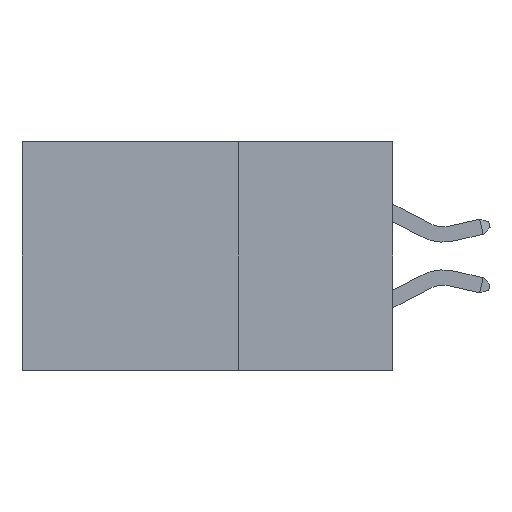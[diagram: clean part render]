
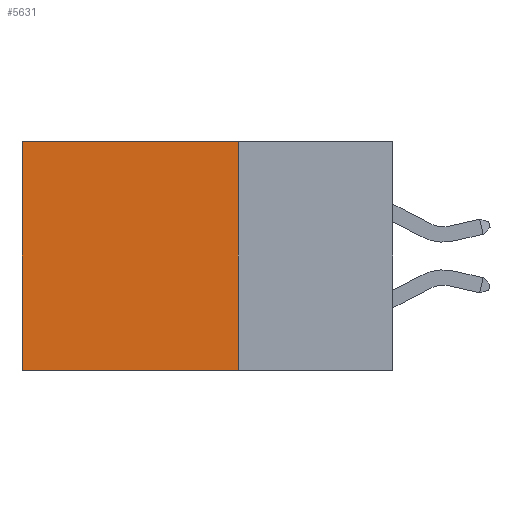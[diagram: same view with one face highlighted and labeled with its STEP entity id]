
A CAD part, left-side view. The second image highlights one B-rep face of the part: STEP entity #5631.
In plain terms, the highlighted planar face has unit normal (-1, 0, 0).
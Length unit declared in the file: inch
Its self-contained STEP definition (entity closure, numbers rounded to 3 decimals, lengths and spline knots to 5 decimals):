
#1334 = VECTOR ( 'NONE', #14771, 39.37008 ) ;
#1614 = LINE ( 'NONE', #5481, #1334 ) ;
#1653 = ORIENTED_EDGE ( 'NONE', *, *, #7843, .T. ) ;
#1659 = EDGE_LOOP ( 'NONE', ( #20980, #11002, #10444, #1653 ) ) ;
#1860 = CARTESIAN_POINT ( 'NONE',  ( 0.2875, 0.6, 0. ) ) ;
#2989 = CARTESIAN_POINT ( 'NONE',  ( 0.2875, 0.25, 0. ) ) ;
#3892 = CARTESIAN_POINT ( 'NONE',  ( 0.2875, 0.6, -0.37 ) ) ;
#5304 = VERTEX_POINT ( 'NONE', #16441 ) ;
#5440 = DIRECTION ( 'NONE',  ( 0., 1., 0. ) ) ;
#5481 = CARTESIAN_POINT ( 'NONE',  ( 0.2875, 0.25, 0. ) ) ;
#5631 = ADVANCED_FACE ( 'NONE', ( #20936 ), #10458, .F. ) ;
#6022 = VECTOR ( 'NONE', #5440, 39.37008 ) ;
#7383 = EDGE_CURVE ( 'NONE', #10903, #13509, #17932, .T. ) ;
#7843 = EDGE_CURVE ( 'NONE', #5304, #9608, #1614, .T. ) ;
#9041 = VECTOR ( 'NONE', #15863, 39.37008 ) ;
#9144 = LINE ( 'NONE', #1860, #16987 ) ;
#9260 = EDGE_CURVE ( 'NONE', #9608, #13509, #9144, .T. ) ;
#9608 = VERTEX_POINT ( 'NONE', #9656 ) ;
#9656 = CARTESIAN_POINT ( 'NONE',  ( 0.2875, 0.6, 0. ) ) ;
#10444 = ORIENTED_EDGE ( 'NONE', *, *, #16003, .F. ) ;
#10458 = PLANE ( 'NONE',  #23147 ) ;
#10541 = DIRECTION ( 'NONE',  ( 0., 0., -1. ) ) ;
#10903 = VERTEX_POINT ( 'NONE', #19038 ) ;
#10960 = CARTESIAN_POINT ( 'NONE',  ( 0.2875, 0.25, -0.37 ) ) ;
#11002 = ORIENTED_EDGE ( 'NONE', *, *, #7383, .F. ) ;
#13509 = VERTEX_POINT ( 'NONE', #3892 ) ;
#14771 = DIRECTION ( 'NONE',  ( 0., 1., 0. ) ) ;
#15863 = DIRECTION ( 'NONE',  ( 0., 0., -1. ) ) ;
#16003 = EDGE_CURVE ( 'NONE', #5304, #10903, #18943, .T. ) ;
#16441 = CARTESIAN_POINT ( 'NONE',  ( 0.2875, 0.25, 0. ) ) ;
#16489 = DIRECTION ( 'NONE',  ( 0., 0., -1. ) ) ;
#16987 = VECTOR ( 'NONE', #16489, 39.37008 ) ;
#17932 = LINE ( 'NONE', #10960, #6022 ) ;
#18943 = LINE ( 'NONE', #21652, #9041 ) ;
#19038 = CARTESIAN_POINT ( 'NONE',  ( 0.2875, 0.25, -0.37 ) ) ;
#19600 = DIRECTION ( 'NONE',  ( 1., 0., 0. ) ) ;
#20936 = FACE_OUTER_BOUND ( 'NONE', #1659, .T. ) ;
#20980 = ORIENTED_EDGE ( 'NONE', *, *, #9260, .T. ) ;
#21652 = CARTESIAN_POINT ( 'NONE',  ( 0.2875, 0.25, 0. ) ) ;
#23147 = AXIS2_PLACEMENT_3D ( 'NONE', #2989, #19600, #10541 ) ;
